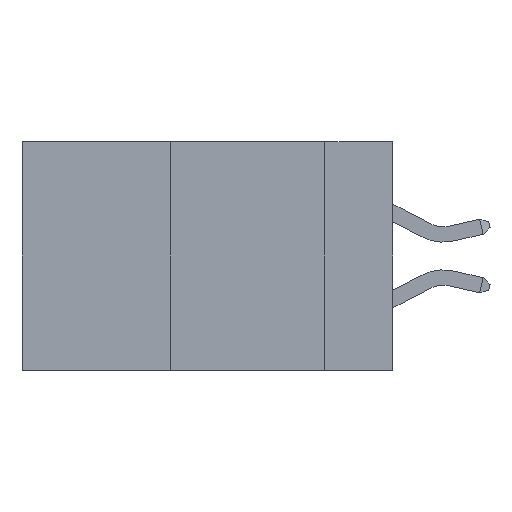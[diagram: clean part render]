
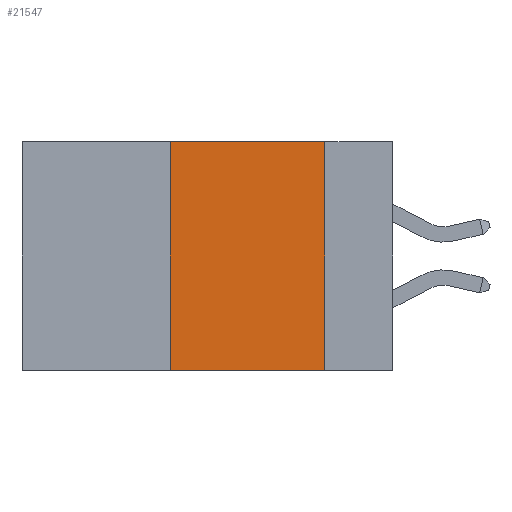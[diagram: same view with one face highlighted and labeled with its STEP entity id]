
A CAD part, left-side view. The second image highlights one B-rep face of the part: STEP entity #21547.
In plain terms, the highlighted planar face has unit normal (-1, 0, 0).
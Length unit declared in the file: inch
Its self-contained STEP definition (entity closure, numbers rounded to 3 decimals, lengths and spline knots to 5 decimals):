
#208 = EDGE_CURVE ( 'NONE', #17074, #11184, #11757, .T. ) ;
#2120 = FACE_OUTER_BOUND ( 'NONE', #7321, .T. ) ;
#2783 = VECTOR ( 'NONE', #13300, 39.37008 ) ;
#3075 = CARTESIAN_POINT ( 'NONE',  ( 0., 0.6, 0. ) ) ;
#3233 = LINE ( 'NONE', #11027, #11661 ) ;
#4773 = DIRECTION ( 'NONE',  ( 0., 0., -1. ) ) ;
#5650 = EDGE_CURVE ( 'NONE', #9968, #17074, #3233, .T. ) ;
#6987 = EDGE_CURVE ( 'NONE', #16869, #11184, #20054, .T. ) ;
#7321 = EDGE_LOOP ( 'NONE', ( #18723, #21060, #19327, #8095 ) ) ;
#7714 = CARTESIAN_POINT ( 'NONE',  ( 0., 0.36, 0. ) ) ;
#8095 = ORIENTED_EDGE ( 'NONE', *, *, #6987, .T. ) ;
#8428 = LINE ( 'NONE', #7714, #12846 ) ;
#8700 = DIRECTION ( 'NONE',  ( 0., -1., 0. ) ) ;
#9968 = VERTEX_POINT ( 'NONE', #13506 ) ;
#10319 = AXIS2_PLACEMENT_3D ( 'NONE', #3075, #14776, #4773 ) ;
#10490 = DIRECTION ( 'NONE',  ( 0., -1., 0. ) ) ;
#11027 = CARTESIAN_POINT ( 'NONE',  ( 0., 0.6, 0. ) ) ;
#11067 = DIRECTION ( 'NONE',  ( 0., 0., 1. ) ) ;
#11184 = VERTEX_POINT ( 'NONE', #14347 ) ;
#11475 = PLANE ( 'NONE',  #10319 ) ;
#11661 = VECTOR ( 'NONE', #10490, 39.37008 ) ;
#11757 = LINE ( 'NONE', #11999, #2783 ) ;
#11802 = EDGE_CURVE ( 'NONE', #16869, #9968, #8428, .T. ) ;
#11895 = VECTOR ( 'NONE', #8700, 39.37008 ) ;
#11999 = CARTESIAN_POINT ( 'NONE',  ( 0., 0.11, 0. ) ) ;
#12286 = CARTESIAN_POINT ( 'NONE',  ( 0., 0.11, 0. ) ) ;
#12846 = VECTOR ( 'NONE', #11067, 39.37008 ) ;
#13300 = DIRECTION ( 'NONE',  ( 0., 0., -1. ) ) ;
#13506 = CARTESIAN_POINT ( 'NONE',  ( 0., 0.36, 0. ) ) ;
#14347 = CARTESIAN_POINT ( 'NONE',  ( 0., 0.11, -0.37 ) ) ;
#14776 = DIRECTION ( 'NONE',  ( 1., 0., 0. ) ) ;
#16736 = CARTESIAN_POINT ( 'NONE',  ( 0., 0.36, -0.37 ) ) ;
#16869 = VERTEX_POINT ( 'NONE', #16736 ) ;
#17074 = VERTEX_POINT ( 'NONE', #12286 ) ;
#18723 = ORIENTED_EDGE ( 'NONE', *, *, #208, .F. ) ;
#19327 = ORIENTED_EDGE ( 'NONE', *, *, #11802, .F. ) ;
#19461 = CARTESIAN_POINT ( 'NONE',  ( 0., 0.6, -0.37 ) ) ;
#20054 = LINE ( 'NONE', #19461, #11895 ) ;
#21060 = ORIENTED_EDGE ( 'NONE', *, *, #5650, .F. ) ;
#21547 = ADVANCED_FACE ( 'NONE', ( #2120 ), #11475, .F. ) ;
